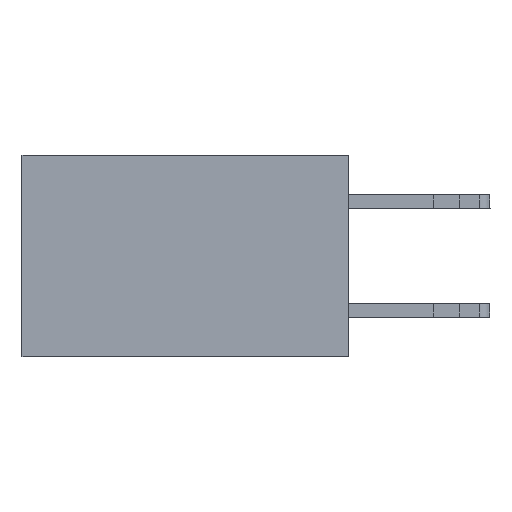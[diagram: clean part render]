
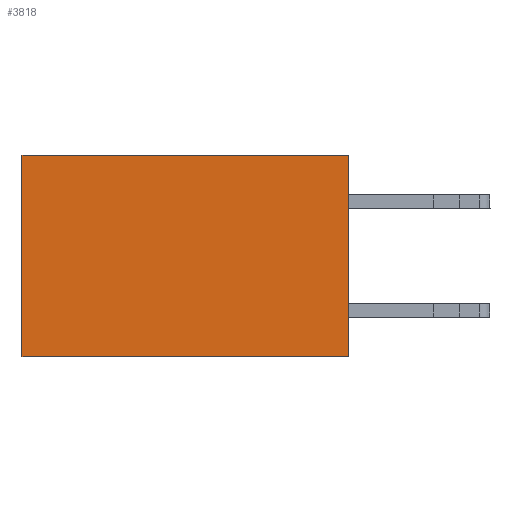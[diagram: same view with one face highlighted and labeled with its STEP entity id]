
A CAD part, left-side view. The second image highlights one B-rep face of the part: STEP entity #3818.
In plain terms, the highlighted planar face has unit normal (-1, 0, 0).
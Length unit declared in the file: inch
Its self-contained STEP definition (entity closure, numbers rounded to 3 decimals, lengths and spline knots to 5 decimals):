
#385 = CARTESIAN_POINT ( 'NONE',  ( 0.2615, 0.6, -0.37 ) ) ;
#618 = EDGE_CURVE ( 'NONE', #16152, #15166, #18368, .T. ) ;
#1746 = DIRECTION ( 'NONE',  ( 0., 0., -1. ) ) ;
#2856 = EDGE_CURVE ( 'NONE', #13958, #16152, #18329, .T. ) ;
#3654 = VECTOR ( 'NONE', #6958, 39.37008 ) ;
#3818 = ADVANCED_FACE ( 'NONE', ( #14797 ), #16383, .F. ) ;
#4483 = EDGE_CURVE ( 'NONE', #10535, #15166, #18833, .T. ) ;
#4712 = ORIENTED_EDGE ( 'NONE', *, *, #2856, .F. ) ;
#5126 = EDGE_LOOP ( 'NONE', ( #11310, #6402, #4712, #13961 ) ) ;
#5568 = CARTESIAN_POINT ( 'NONE',  ( 0.2615, 0., 0. ) ) ;
#6402 = ORIENTED_EDGE ( 'NONE', *, *, #618, .F. ) ;
#6476 = CARTESIAN_POINT ( 'NONE',  ( 0.2615, 0., -0.37 ) ) ;
#6958 = DIRECTION ( 'NONE',  ( 0., 1., 0. ) ) ;
#7437 = VECTOR ( 'NONE', #8650, 39.37008 ) ;
#7559 = VECTOR ( 'NONE', #10865, 39.37008 ) ;
#7635 = AXIS2_PLACEMENT_3D ( 'NONE', #9087, #13518, #12027 ) ;
#8216 = VECTOR ( 'NONE', #1746, 39.37008 ) ;
#8650 = DIRECTION ( 'NONE',  ( 0., 0., -1. ) ) ;
#9087 = CARTESIAN_POINT ( 'NONE',  ( 0.2615, 0., -0.37 ) ) ;
#9186 = EDGE_CURVE ( 'NONE', #13958, #10535, #19013, .T. ) ;
#9923 = CARTESIAN_POINT ( 'NONE',  ( 0.2615, 0.6, -0.37 ) ) ;
#10535 = VERTEX_POINT ( 'NONE', #14381 ) ;
#10865 = DIRECTION ( 'NONE',  ( 0., 1., 0. ) ) ;
#11310 = ORIENTED_EDGE ( 'NONE', *, *, #4483, .T. ) ;
#12007 = CARTESIAN_POINT ( 'NONE',  ( 0.2615, 0., 0. ) ) ;
#12027 = DIRECTION ( 'NONE',  ( 0., 0., -1. ) ) ;
#12738 = CARTESIAN_POINT ( 'NONE',  ( 0.2615, 0., -0.37 ) ) ;
#13518 = DIRECTION ( 'NONE',  ( 1., 0., 0. ) ) ;
#13958 = VERTEX_POINT ( 'NONE', #12007 ) ;
#13961 = ORIENTED_EDGE ( 'NONE', *, *, #9186, .T. ) ;
#14381 = CARTESIAN_POINT ( 'NONE',  ( 0.2615, 0.6, 0. ) ) ;
#14797 = FACE_OUTER_BOUND ( 'NONE', #5126, .T. ) ;
#15166 = VERTEX_POINT ( 'NONE', #385 ) ;
#16152 = VERTEX_POINT ( 'NONE', #12738 ) ;
#16383 = PLANE ( 'NONE',  #7635 ) ;
#17088 = CARTESIAN_POINT ( 'NONE',  ( 0.2615, 0., -0.37 ) ) ;
#18329 = LINE ( 'NONE', #6476, #8216 ) ;
#18368 = LINE ( 'NONE', #17088, #7559 ) ;
#18833 = LINE ( 'NONE', #9923, #7437 ) ;
#19013 = LINE ( 'NONE', #5568, #3654 ) ;
